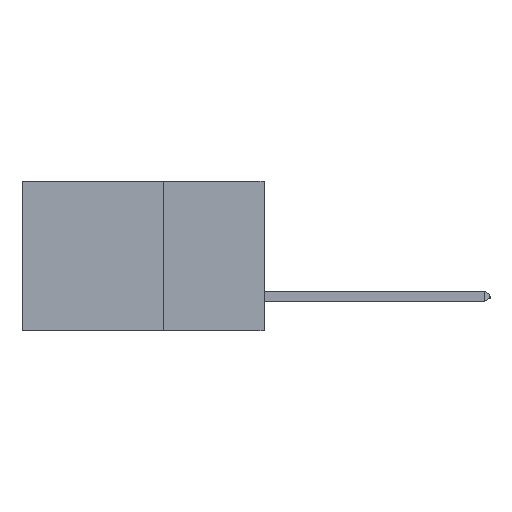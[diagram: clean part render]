
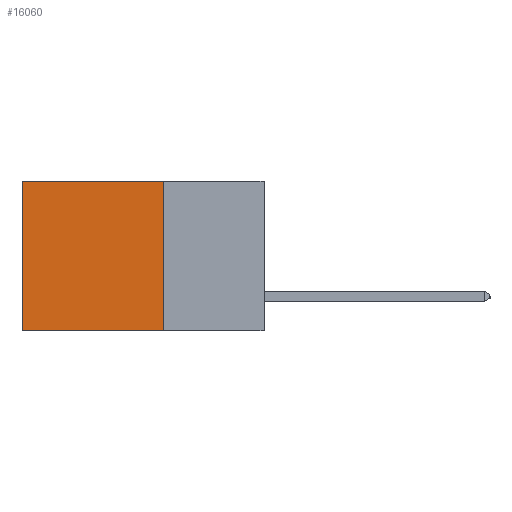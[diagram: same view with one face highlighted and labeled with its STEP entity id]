
A CAD part, left-side view. The second image highlights one B-rep face of the part: STEP entity #16060.
In plain terms, the highlighted planar face has unit normal (-1, 0, 0).
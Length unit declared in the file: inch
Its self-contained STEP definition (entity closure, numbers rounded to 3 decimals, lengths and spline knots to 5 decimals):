
#76 = DIRECTION ( 'NONE',  ( 0., 0., -1. ) ) ;
#691 = EDGE_CURVE ( 'NONE', #11556, #11411, #2161, .T. ) ;
#1189 = CARTESIAN_POINT ( 'NONE',  ( 0.298, 0.25, 0. ) ) ;
#1232 = LINE ( 'NONE', #15194, #11466 ) ;
#2061 = EDGE_LOOP ( 'NONE', ( #16325, #2923, #3831, #5908 ) ) ;
#2161 = LINE ( 'NONE', #16009, #15676 ) ;
#2219 = CARTESIAN_POINT ( 'NONE',  ( 0.298, 0.25, -0.37 ) ) ;
#2569 = VECTOR ( 'NONE', #13826, 39.37008 ) ;
#2923 = ORIENTED_EDGE ( 'NONE', *, *, #9568, .F. ) ;
#3183 = DIRECTION ( 'NONE',  ( 1., 0., 0. ) ) ;
#3340 = VERTEX_POINT ( 'NONE', #5346 ) ;
#3831 = ORIENTED_EDGE ( 'NONE', *, *, #691, .F. ) ;
#3988 = LINE ( 'NONE', #15878, #10656 ) ;
#4230 = VERTEX_POINT ( 'NONE', #7072 ) ;
#4772 = CARTESIAN_POINT ( 'NONE',  ( 0.298, 0.25, 0. ) ) ;
#5346 = CARTESIAN_POINT ( 'NONE',  ( 0.298, 0.6, -0.37 ) ) ;
#5893 = PLANE ( 'NONE',  #8400 ) ;
#5908 = ORIENTED_EDGE ( 'NONE', *, *, #7588, .T. ) ;
#6209 = LINE ( 'NONE', #4772, #2569 ) ;
#6259 = FACE_OUTER_BOUND ( 'NONE', #2061, .T. ) ;
#7072 = CARTESIAN_POINT ( 'NONE',  ( 0.298, 0.6, 0. ) ) ;
#7588 = EDGE_CURVE ( 'NONE', #11556, #4230, #6209, .T. ) ;
#8400 = AXIS2_PLACEMENT_3D ( 'NONE', #11157, #3183, #12449 ) ;
#9568 = EDGE_CURVE ( 'NONE', #11411, #3340, #1232, .T. ) ;
#10656 = VECTOR ( 'NONE', #76, 39.37008 ) ;
#11157 = CARTESIAN_POINT ( 'NONE',  ( 0.298, 0.25, 0. ) ) ;
#11383 = DIRECTION ( 'NONE',  ( 0., 1., 0. ) ) ;
#11411 = VERTEX_POINT ( 'NONE', #2219 ) ;
#11466 = VECTOR ( 'NONE', #11383, 39.37008 ) ;
#11556 = VERTEX_POINT ( 'NONE', #1189 ) ;
#12449 = DIRECTION ( 'NONE',  ( 0., 0., -1. ) ) ;
#12625 = DIRECTION ( 'NONE',  ( 0., 0., -1. ) ) ;
#13433 = EDGE_CURVE ( 'NONE', #4230, #3340, #3988, .T. ) ;
#13826 = DIRECTION ( 'NONE',  ( 0., 1., 0. ) ) ;
#15194 = CARTESIAN_POINT ( 'NONE',  ( 0.298, 0.25, -0.37 ) ) ;
#15676 = VECTOR ( 'NONE', #12625, 39.37008 ) ;
#15878 = CARTESIAN_POINT ( 'NONE',  ( 0.298, 0.6, 0. ) ) ;
#16009 = CARTESIAN_POINT ( 'NONE',  ( 0.298, 0.25, 0. ) ) ;
#16060 = ADVANCED_FACE ( 'NONE', ( #6259 ), #5893, .F. ) ;
#16325 = ORIENTED_EDGE ( 'NONE', *, *, #13433, .T. ) ;
